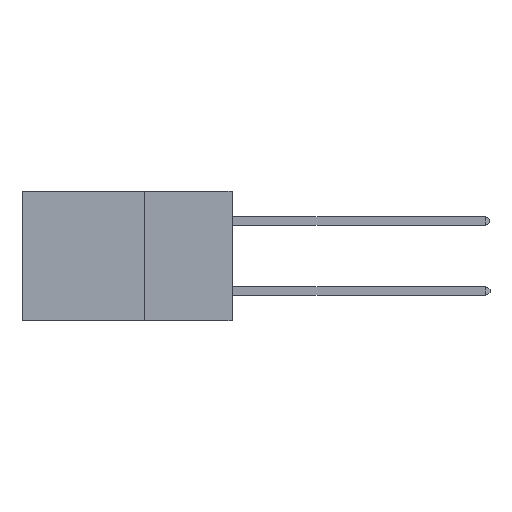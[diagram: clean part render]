
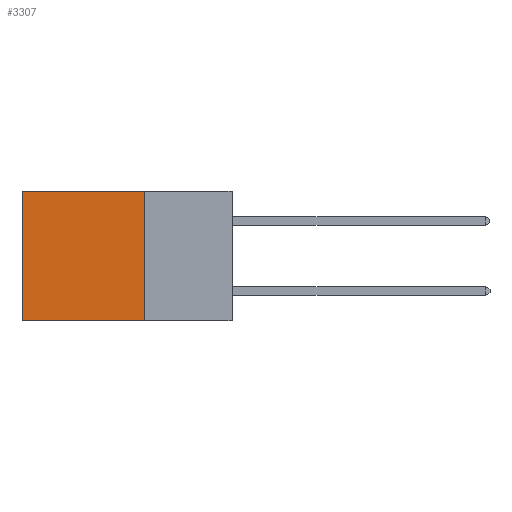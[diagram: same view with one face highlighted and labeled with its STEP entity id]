
A CAD part, left-side view. The second image highlights one B-rep face of the part: STEP entity #3307.
In plain terms, the highlighted planar face has unit normal (-1, 0, 0).
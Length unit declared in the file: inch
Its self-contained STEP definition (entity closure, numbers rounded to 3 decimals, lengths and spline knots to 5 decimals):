
#456 = AXIS2_PLACEMENT_3D ( 'NONE', #2736, #2439, #2436 ) ;
#957 = VERTEX_POINT ( 'NONE', #8603 ) ;
#1446 = LINE ( 'NONE', #18580, #9992 ) ;
#1697 = DIRECTION ( 'NONE',  ( 0., 1., 0. ) ) ;
#2301 = VECTOR ( 'NONE', #8859, 39.37008 ) ;
#2436 = DIRECTION ( 'NONE',  ( 0., 0., -1. ) ) ;
#2439 = DIRECTION ( 'NONE',  ( 1., 0., 0. ) ) ;
#2462 = PLANE ( 'NONE',  #456 ) ;
#2736 = CARTESIAN_POINT ( 'NONE',  ( 0.2875, 0.25, 0. ) ) ;
#3307 = ADVANCED_FACE ( 'NONE', ( #20055 ), #2462, .F. ) ;
#5404 = ORIENTED_EDGE ( 'NONE', *, *, #13959, .T. ) ;
#5990 = VERTEX_POINT ( 'NONE', #6126 ) ;
#6027 = VECTOR ( 'NONE', #21329, 39.37008 ) ;
#6104 = ORIENTED_EDGE ( 'NONE', *, *, #15393, .T. ) ;
#6126 = CARTESIAN_POINT ( 'NONE',  ( 0.2875, 0.6, -0.37 ) ) ;
#6552 = LINE ( 'NONE', #16425, #6027 ) ;
#6874 = LINE ( 'NONE', #13846, #2301 ) ;
#7531 = EDGE_LOOP ( 'NONE', ( #5404, #20090, #16671, #6104 ) ) ;
#8199 = VERTEX_POINT ( 'NONE', #20479 ) ;
#8603 = CARTESIAN_POINT ( 'NONE',  ( 0.2875, 0.25, -0.37 ) ) ;
#8859 = DIRECTION ( 'NONE',  ( 0., 0., -1. ) ) ;
#8867 = EDGE_CURVE ( 'NONE', #11711, #957, #6874, .T. ) ;
#9547 = DIRECTION ( 'NONE',  ( 0., 0., -1. ) ) ;
#9992 = VECTOR ( 'NONE', #1697, 39.37008 ) ;
#11711 = VERTEX_POINT ( 'NONE', #19835 ) ;
#11911 = CARTESIAN_POINT ( 'NONE',  ( 0.2875, 0.6, 0. ) ) ;
#13846 = CARTESIAN_POINT ( 'NONE',  ( 0.2875, 0.25, 0. ) ) ;
#13959 = EDGE_CURVE ( 'NONE', #8199, #5990, #20715, .T. ) ;
#14951 = EDGE_CURVE ( 'NONE', #957, #5990, #6552, .T. ) ;
#15393 = EDGE_CURVE ( 'NONE', #11711, #8199, #1446, .T. ) ;
#16401 = VECTOR ( 'NONE', #9547, 39.37008 ) ;
#16425 = CARTESIAN_POINT ( 'NONE',  ( 0.2875, 0.25, -0.37 ) ) ;
#16671 = ORIENTED_EDGE ( 'NONE', *, *, #8867, .F. ) ;
#18580 = CARTESIAN_POINT ( 'NONE',  ( 0.2875, 0.25, 0. ) ) ;
#19835 = CARTESIAN_POINT ( 'NONE',  ( 0.2875, 0.25, 0. ) ) ;
#20055 = FACE_OUTER_BOUND ( 'NONE', #7531, .T. ) ;
#20090 = ORIENTED_EDGE ( 'NONE', *, *, #14951, .F. ) ;
#20479 = CARTESIAN_POINT ( 'NONE',  ( 0.2875, 0.6, 0. ) ) ;
#20715 = LINE ( 'NONE', #11911, #16401 ) ;
#21329 = DIRECTION ( 'NONE',  ( 0., 1., 0. ) ) ;
